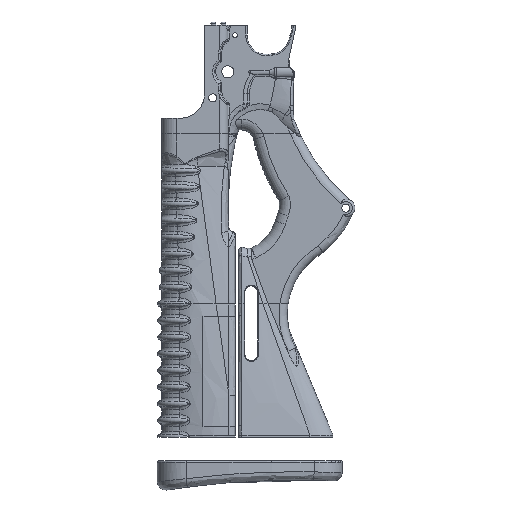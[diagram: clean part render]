
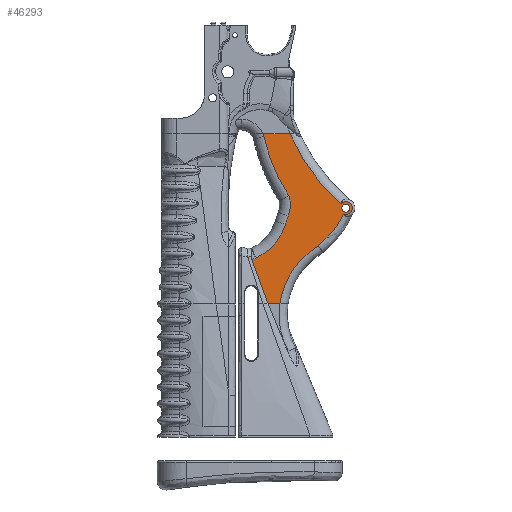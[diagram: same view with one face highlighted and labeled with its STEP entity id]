
A CAD part, front view. The second image highlights one B-rep face of the part: STEP entity #46293.
In plain terms, the highlighted planar face has unit normal (0, -1, 0).
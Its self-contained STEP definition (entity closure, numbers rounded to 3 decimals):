
#2886=B_SPLINE_CURVE_WITH_KNOTS('',3,(#121153,#121154,#121155,#121156),
 .UNSPECIFIED.,.F.,.F.,(4,4),(0.414,4.122),
 .UNSPECIFIED.);
#2887=B_SPLINE_CURVE_WITH_KNOTS('',3,(#121162,#121163,#121164,#121165),
 .UNSPECIFIED.,.F.,.F.,(4,4),(2.914,2.915),
 .UNSPECIFIED.);
#4070=FACE_BOUND('',#9548,.T.);
#4928=PLANE('',#49176);
#6783=FACE_OUTER_BOUND('',#9547,.T.);
#9547=EDGE_LOOP('',(#38772,#38773,#38774,#38775,#38776,#38777,#38778,#38779,
#38780,#38781,#38782,#38783,#38784,#38785,#38786));
#9548=EDGE_LOOP('',(#38787));
#12761=LINE('',#121137,#15674);
#12762=LINE('',#121151,#15675);
#12763=LINE('',#121158,#15676);
#15674=VECTOR('',#56415,10.);
#15675=VECTOR('',#56428,10.);
#15676=VECTOR('',#56429,10.);
#17142=CIRCLE('',#49171,5.08);
#17145=CIRCLE('',#49177,153.137);
#17146=CIRCLE('',#49178,19.266);
#17147=CIRCLE('',#49179,144.127);
#17148=CIRCLE('',#49180,24.878);
#17149=CIRCLE('',#49181,124.5);
#17150=CIRCLE('',#49182,43.01);
#17151=CIRCLE('',#49183,8.5);
#17152=CIRCLE('',#49184,62.91);
#17153=CIRCLE('',#49185,66.451);
#17154=CIRCLE('',#49186,3.175);
#20885=VERTEX_POINT('',#120999);
#20888=VERTEX_POINT('',#121017);
#20899=VERTEX_POINT('',#121134);
#20900=VERTEX_POINT('',#121136);
#20901=VERTEX_POINT('',#121138);
#20902=VERTEX_POINT('',#121140);
#20903=VERTEX_POINT('',#121142);
#20904=VERTEX_POINT('',#121144);
#20905=VERTEX_POINT('',#121146);
#20906=VERTEX_POINT('',#121148);
#20907=VERTEX_POINT('',#121150);
#20908=VERTEX_POINT('',#121152);
#20909=VERTEX_POINT('',#121157);
#20910=VERTEX_POINT('',#121159);
#20911=VERTEX_POINT('',#121161);
#20912=VERTEX_POINT('',#121167);
#27091=EDGE_CURVE('',#20888,#20885,#17142,.T.);
#27104=EDGE_CURVE('',#20899,#20888,#17145,.T.);
#27105=EDGE_CURVE('',#20899,#20900,#12761,.T.);
#27106=EDGE_CURVE('',#20901,#20900,#17146,.T.);
#27107=EDGE_CURVE('',#20902,#20901,#17147,.T.);
#27108=EDGE_CURVE('',#20903,#20902,#17148,.T.);
#27109=EDGE_CURVE('',#20904,#20903,#17149,.T.);
#27110=EDGE_CURVE('',#20905,#20904,#17150,.T.);
#27111=EDGE_CURVE('',#20906,#20905,#17151,.T.);
#27112=EDGE_CURVE('',#20907,#20906,#12762,.T.);
#27113=EDGE_CURVE('',#20907,#20908,#2886,.T.);
#27114=EDGE_CURVE('',#20908,#20909,#12763,.T.);
#27115=EDGE_CURVE('',#20910,#20909,#17152,.T.);
#27116=EDGE_CURVE('',#20911,#20910,#2887,.T.);
#27117=EDGE_CURVE('',#20885,#20911,#17153,.T.);
#27118=EDGE_CURVE('',#20912,#20912,#17154,.T.);
#38772=ORIENTED_EDGE('',*,*,#27104,.F.);
#38773=ORIENTED_EDGE('',*,*,#27105,.T.);
#38774=ORIENTED_EDGE('',*,*,#27106,.F.);
#38775=ORIENTED_EDGE('',*,*,#27107,.F.);
#38776=ORIENTED_EDGE('',*,*,#27108,.F.);
#38777=ORIENTED_EDGE('',*,*,#27109,.F.);
#38778=ORIENTED_EDGE('',*,*,#27110,.F.);
#38779=ORIENTED_EDGE('',*,*,#27111,.F.);
#38780=ORIENTED_EDGE('',*,*,#27112,.F.);
#38781=ORIENTED_EDGE('',*,*,#27113,.T.);
#38782=ORIENTED_EDGE('',*,*,#27114,.T.);
#38783=ORIENTED_EDGE('',*,*,#27115,.F.);
#38784=ORIENTED_EDGE('',*,*,#27116,.F.);
#38785=ORIENTED_EDGE('',*,*,#27117,.F.);
#38786=ORIENTED_EDGE('',*,*,#27091,.F.);
#38787=ORIENTED_EDGE('',*,*,#27118,.T.);
#46293=ADVANCED_FACE('',(#6783,#4070),#4928,.T.);
#49171=AXIS2_PLACEMENT_3D('',#121030,#56399,#56400);
#49176=AXIS2_PLACEMENT_3D('',#121133,#56411,#56412);
#49177=AXIS2_PLACEMENT_3D('',#121135,#56413,#56414);
#49178=AXIS2_PLACEMENT_3D('',#121139,#56416,#56417);
#49179=AXIS2_PLACEMENT_3D('',#121141,#56418,#56419);
#49180=AXIS2_PLACEMENT_3D('',#121143,#56420,#56421);
#49181=AXIS2_PLACEMENT_3D('',#121145,#56422,#56423);
#49182=AXIS2_PLACEMENT_3D('',#121147,#56424,#56425);
#49183=AXIS2_PLACEMENT_3D('',#121149,#56426,#56427);
#49184=AXIS2_PLACEMENT_3D('',#121160,#56430,#56431);
#49185=AXIS2_PLACEMENT_3D('',#121166,#56432,#56433);
#49186=AXIS2_PLACEMENT_3D('',#121168,#56434,#56435);
#56399=DIRECTION('center_axis',(0.,1.,0.));
#56400=DIRECTION('ref_axis',(0.974,0.,0.226));
#56411=DIRECTION('center_axis',(0.,-1.,0.));
#56412=DIRECTION('ref_axis',(0.,0.,
1.));
#56413=DIRECTION('center_axis',(0.,-1.,0.));
#56414=DIRECTION('ref_axis',(-0.782,0.,-0.624));
#56415=DIRECTION('',(-1.,0.,0.));
#56416=DIRECTION('center_axis',(0.,-1.,0.));
#56417=DIRECTION('ref_axis',(0.619,0.,0.785));
#56418=DIRECTION('center_axis',(0.,1.,0.));
#56419=DIRECTION('ref_axis',(-0.923,0.,-0.385));
#56420=DIRECTION('center_axis',(0.,-1.,0.));
#56421=DIRECTION('ref_axis',(0.986,0.,-0.164));
#56422=DIRECTION('center_axis',(0.,1.,0.));
#56423=DIRECTION('ref_axis',(-0.946,0.,0.323));
#56424=DIRECTION('center_axis',(0.,-1.,0.));
#56425=DIRECTION('ref_axis',(0.792,0.,-0.61));
#56426=DIRECTION('center_axis',(0.,-1.,0.));
#56427=DIRECTION('ref_axis',(-0.423,0.,0.906));
#56428=DIRECTION('',(0.95,0.,0.312));
#56429=DIRECTION('',(1.,0.,0.));
#56430=DIRECTION('center_axis',(0.,-1.,0.));
#56431=DIRECTION('ref_axis',(-0.955,0.,0.295));
#56432=DIRECTION('center_axis',(0.,1.,0.));
#56433=DIRECTION('ref_axis',(0.796,0.,-0.606));
#56434=DIRECTION('center_axis',(0.,1.,0.));
#56435=DIRECTION('ref_axis',(0.,0.,
1.));
#120999=CARTESIAN_POINT('',(83.21,-20.163,-164.8));
#121017=CARTESIAN_POINT('',(81.266,-20.163,-156.815));
#121030=CARTESIAN_POINT('Origin',(85.14,-20.163,-160.101));
#121133=CARTESIAN_POINT('Origin',(29.836,-20.163,-156.541));
#121134=CARTESIAN_POINT('',(41.472,-20.163,-101.96));
#121135=CARTESIAN_POINT('Origin',(182.252,-20.163,-41.695));
#121136=CARTESIAN_POINT('',(20.214,-20.163,-101.96));
#121137=CARTESIAN_POINT('',(21.855,-20.163,-101.96));
#121138=CARTESIAN_POINT('',(20.963,-20.163,-103.985));
#121139=CARTESIAN_POINT('Origin',(2.546,-20.163,-109.642));
#121140=CARTESIAN_POINT('',(40.643,-20.163,-150.775));
#121141=CARTESIAN_POINT('Origin',(161.581,-20.163,-72.374));
#121142=CARTESIAN_POINT('',(40.068,-20.163,-166.399));
#121143=CARTESIAN_POINT('Origin',(16.753,-20.163,-157.719));
#121144=CARTESIAN_POINT('',(37.861,-20.163,-172.864));
#121145=CARTESIAN_POINT('Origin',(156.744,-20.163,-209.837));
#121146=CARTESIAN_POINT('',(14.989,-20.163,-199.062));
#121147=CARTESIAN_POINT('Origin',(-3.208,-20.163,-160.092));
#121148=CARTESIAN_POINT('',(14.043,-20.163,-199.437));
#121149=CARTESIAN_POINT('Origin',(11.393,-20.163,-191.36));
#121150=CARTESIAN_POINT('',(11.444,-20.163,-200.29));
#121151=CARTESIAN_POINT('',(27.525,-20.163,-195.013));
#121152=CARTESIAN_POINT('',(24.214,-20.163,-235.143));
#121153=CARTESIAN_POINT('Ctrl Pts',(11.444,-20.163,
-200.29));
#121154=CARTESIAN_POINT('Ctrl Pts',(15.408,-20.163,
-211.999));
#121155=CARTESIAN_POINT('Ctrl Pts',(19.706,-20.163,
-223.61));
#121156=CARTESIAN_POINT('Ctrl Pts',(24.214,-20.163,
-235.143));
#121157=CARTESIAN_POINT('',(33.422,-20.163,-235.143));
#121158=CARTESIAN_POINT('',(32.181,-20.163,-235.143));
#121159=CARTESIAN_POINT('',(63.128,-20.163,-189.989));
#121160=CARTESIAN_POINT('Origin',(95.734,-20.163,-243.789));
#121161=CARTESIAN_POINT('',(63.134,-20.163,-189.993));
#121162=CARTESIAN_POINT('Ctrl Pts',(63.134,-20.163,
-189.993));
#121163=CARTESIAN_POINT('Ctrl Pts',(63.132,-20.163,
-189.992));
#121164=CARTESIAN_POINT('Ctrl Pts',(63.13,-20.163,
-189.991));
#121165=CARTESIAN_POINT('Ctrl Pts',(63.128,-20.163,
-189.989));
#121166=CARTESIAN_POINT('Origin',(22.753,-20.163,-137.219));
#121167=CARTESIAN_POINT('',(85.14,-20.163,-163.276));
#121168=CARTESIAN_POINT('Origin',(85.14,-20.163,-160.101));
